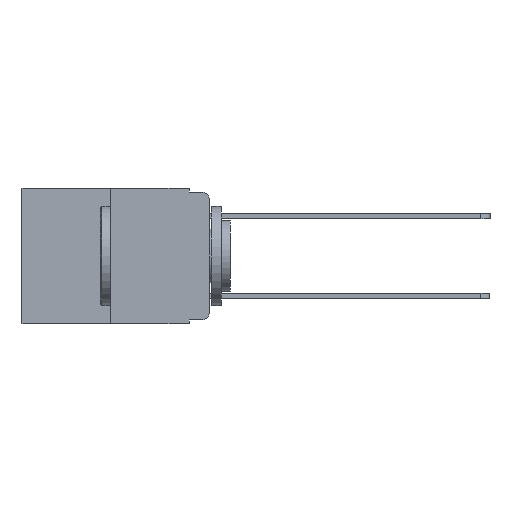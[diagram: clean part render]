
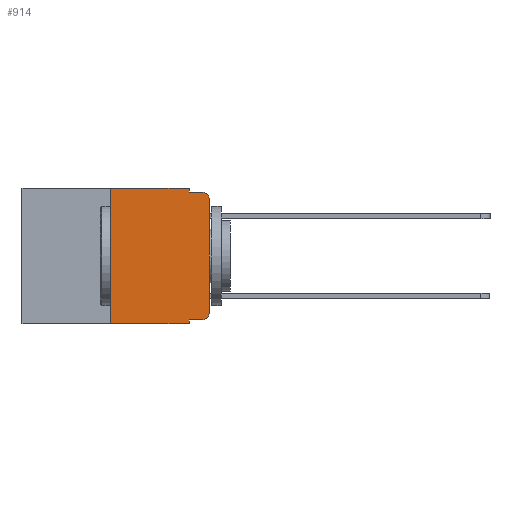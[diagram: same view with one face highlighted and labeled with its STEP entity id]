
A CAD part, left-side view. The second image highlights one B-rep face of the part: STEP entity #914.
In plain terms, the highlighted planar face has unit normal (-1, 0, 0).
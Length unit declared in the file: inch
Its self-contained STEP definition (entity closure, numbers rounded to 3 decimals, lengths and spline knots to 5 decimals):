
#226 = VECTOR ( 'NONE', #8490, 39.37008 ) ;
#358 = CARTESIAN_POINT ( 'NONE',  ( 0., 0.051, -0.333 ) ) ;
#395 = PLANE ( 'NONE',  #2683 ) ;
#531 = CARTESIAN_POINT ( 'NONE',  ( 0., 0.25, 0. ) ) ;
#544 = CARTESIAN_POINT ( 'NONE',  ( 0., 0.473, 0. ) ) ;
#580 = EDGE_CURVE ( 'NONE', #4128, #854, #5564, .T. ) ;
#801 = VERTEX_POINT ( 'NONE', #358 ) ;
#854 = VERTEX_POINT ( 'NONE', #13952 ) ;
#887 = CARTESIAN_POINT ( 'NONE',  ( 0., 0.051, -0.01 ) ) ;
#914 = ADVANCED_FACE ( 'NONE', ( #7270 ), #395, .F. ) ;
#955 = VERTEX_POINT ( 'NONE', #887 ) ;
#1446 = EDGE_CURVE ( 'NONE', #801, #4128, #8106, .T. ) ;
#1623 = DIRECTION ( 'NONE',  ( 0., -1., 0. ) ) ;
#1638 = CARTESIAN_POINT ( 'NONE',  ( 0., 0.051, -0.333 ) ) ;
#1721 = CARTESIAN_POINT ( 'NONE',  ( 0., 0.25, -0.343 ) ) ;
#1789 = DIRECTION ( 'NONE',  ( 0., 0., -1. ) ) ;
#1825 = VECTOR ( 'NONE', #6367, 39.37008 ) ;
#1862 = DIRECTION ( 'NONE',  ( 1., 0., 0. ) ) ;
#2093 = ORIENTED_EDGE ( 'NONE', *, *, #2978, .F. ) ;
#2200 = EDGE_CURVE ( 'NONE', #801, #10110, #7923, .T. ) ;
#2415 = EDGE_CURVE ( 'NONE', #4507, #10110, #13847, .T. ) ;
#2683 = AXIS2_PLACEMENT_3D ( 'NONE', #544, #1862, #1789 ) ;
#2696 = DIRECTION ( 'NONE',  ( 0., -1., 0. ) ) ;
#2978 = EDGE_CURVE ( 'NONE', #4507, #6579, #5663, .T. ) ;
#3358 = CARTESIAN_POINT ( 'NONE',  ( 0., 0.02, -0.03 ) ) ;
#3409 = ORIENTED_EDGE ( 'NONE', *, *, #6847, .F. ) ;
#3645 = VERTEX_POINT ( 'NONE', #12145 ) ;
#3784 = VERTEX_POINT ( 'NONE', #4774 ) ;
#3804 = LINE ( 'NONE', #10631, #226 ) ;
#3976 = VECTOR ( 'NONE', #12927, 39.37008 ) ;
#4128 = VERTEX_POINT ( 'NONE', #8102 ) ;
#4347 = LINE ( 'NONE', #8913, #3976 ) ;
#4507 = VERTEX_POINT ( 'NONE', #1721 ) ;
#4564 = DIRECTION ( 'NONE',  ( 0., 0., -1. ) ) ;
#4607 = EDGE_CURVE ( 'NONE', #3645, #955, #3804, .T. ) ;
#4774 = CARTESIAN_POINT ( 'NONE',  ( 0., 0., -0.03 ) ) ;
#5195 = VECTOR ( 'NONE', #1623, 39.37008 ) ;
#5418 = LINE ( 'NONE', #7245, #13439 ) ;
#5564 = CIRCLE ( 'NONE', #8551, 0.02 ) ;
#5661 = CARTESIAN_POINT ( 'NONE',  ( 0., 0.473, -0.343 ) ) ;
#5663 = LINE ( 'NONE', #531, #10970 ) ;
#5686 = DIRECTION ( 'NONE',  ( 0., -1., 0. ) ) ;
#5785 = AXIS2_PLACEMENT_3D ( 'NONE', #3358, #10978, #4564 ) ;
#6253 = CARTESIAN_POINT ( 'NONE',  ( 0., 0.051, 0. ) ) ;
#6367 = DIRECTION ( 'NONE',  ( 0., 0., -1. ) ) ;
#6579 = VERTEX_POINT ( 'NONE', #11444 ) ;
#6847 = EDGE_CURVE ( 'NONE', #955, #6932, #4347, .T. ) ;
#6932 = VERTEX_POINT ( 'NONE', #9001 ) ;
#7226 = EDGE_CURVE ( 'NONE', #6579, #3645, #5418, .T. ) ;
#7245 = CARTESIAN_POINT ( 'NONE',  ( 0., 0.473, 0. ) ) ;
#7270 = FACE_OUTER_BOUND ( 'NONE', #7485, .T. ) ;
#7485 = EDGE_LOOP ( 'NONE', ( #7612, #10553, #3409, #9168, #11820, #2093, #12136, #9320, #10909, #12324 ) ) ;
#7565 = EDGE_CURVE ( 'NONE', #3784, #6932, #8989, .T. ) ;
#7575 = CARTESIAN_POINT ( 'NONE',  ( 0., 0., 0. ) ) ;
#7612 = ORIENTED_EDGE ( 'NONE', *, *, #8295, .T. ) ;
#7923 = LINE ( 'NONE', #6253, #1825 ) ;
#8102 = CARTESIAN_POINT ( 'NONE',  ( 0., 0.02, -0.333 ) ) ;
#8106 = LINE ( 'NONE', #1638, #5195 ) ;
#8295 = EDGE_CURVE ( 'NONE', #854, #3784, #12684, .T. ) ;
#8490 = DIRECTION ( 'NONE',  ( 0., 0., -1. ) ) ;
#8551 = AXIS2_PLACEMENT_3D ( 'NONE', #13352, #13320, #13158 ) ;
#8913 = CARTESIAN_POINT ( 'NONE',  ( 0., 0.051, -0.01 ) ) ;
#8989 = CIRCLE ( 'NONE', #5785, 0.02 ) ;
#9001 = CARTESIAN_POINT ( 'NONE',  ( 0., 0.02, -0.01 ) ) ;
#9168 = ORIENTED_EDGE ( 'NONE', *, *, #4607, .F. ) ;
#9320 = ORIENTED_EDGE ( 'NONE', *, *, #2200, .F. ) ;
#10019 = VECTOR ( 'NONE', #12658, 39.37008 ) ;
#10110 = VERTEX_POINT ( 'NONE', #12019 ) ;
#10370 = DIRECTION ( 'NONE',  ( 0., 0., 1. ) ) ;
#10553 = ORIENTED_EDGE ( 'NONE', *, *, #7565, .T. ) ;
#10631 = CARTESIAN_POINT ( 'NONE',  ( 0., 0.051, 0. ) ) ;
#10909 = ORIENTED_EDGE ( 'NONE', *, *, #1446, .T. ) ;
#10970 = VECTOR ( 'NONE', #10370, 39.37008 ) ;
#10978 = DIRECTION ( 'NONE',  ( -1., 0., 0. ) ) ;
#11139 = VECTOR ( 'NONE', #5686, 39.37008 ) ;
#11444 = CARTESIAN_POINT ( 'NONE',  ( 0., 0.25, 0. ) ) ;
#11820 = ORIENTED_EDGE ( 'NONE', *, *, #7226, .F. ) ;
#12019 = CARTESIAN_POINT ( 'NONE',  ( 0., 0.051, -0.343 ) ) ;
#12136 = ORIENTED_EDGE ( 'NONE', *, *, #2415, .T. ) ;
#12145 = CARTESIAN_POINT ( 'NONE',  ( 0., 0.051, 0. ) ) ;
#12324 = ORIENTED_EDGE ( 'NONE', *, *, #580, .T. ) ;
#12658 = DIRECTION ( 'NONE',  ( 0., 0., 1. ) ) ;
#12684 = LINE ( 'NONE', #7575, #10019 ) ;
#12927 = DIRECTION ( 'NONE',  ( 0., -1., 0. ) ) ;
#13158 = DIRECTION ( 'NONE',  ( 0., 0., -1. ) ) ;
#13320 = DIRECTION ( 'NONE',  ( -1., 0., 0. ) ) ;
#13352 = CARTESIAN_POINT ( 'NONE',  ( 0., 0.02, -0.313 ) ) ;
#13439 = VECTOR ( 'NONE', #2696, 39.37008 ) ;
#13847 = LINE ( 'NONE', #5661, #11139 ) ;
#13952 = CARTESIAN_POINT ( 'NONE',  ( 0., 0., -0.313 ) ) ;
